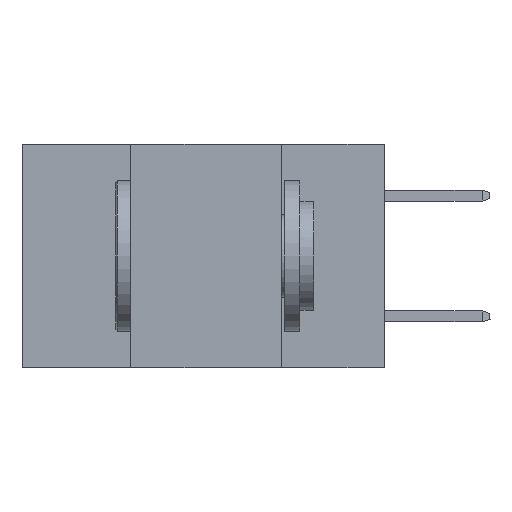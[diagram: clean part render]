
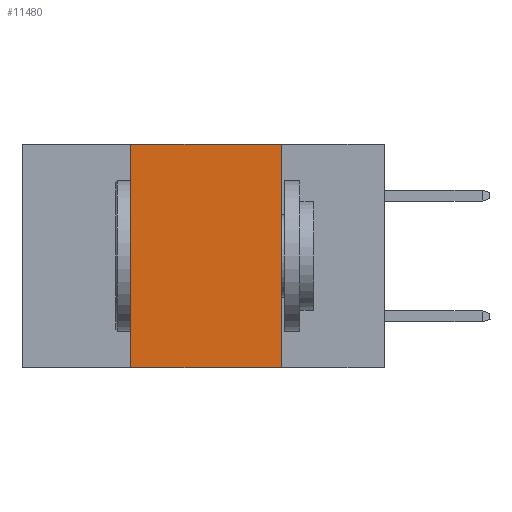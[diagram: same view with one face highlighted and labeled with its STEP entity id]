
A CAD part, left-side view. The second image highlights one B-rep face of the part: STEP entity #11480.
In plain terms, the highlighted planar face has unit normal (-1, 0, 0).
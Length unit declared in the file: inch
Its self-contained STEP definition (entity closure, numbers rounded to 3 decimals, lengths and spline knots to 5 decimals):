
#201 = CARTESIAN_POINT ( 'NONE',  ( 0., 0.17, -0.37 ) ) ;
#339 = AXIS2_PLACEMENT_3D ( 'NONE', #7886, #878, #10653 ) ;
#878 = DIRECTION ( 'NONE',  ( 1., 0., 0. ) ) ;
#1037 = CARTESIAN_POINT ( 'NONE',  ( 0., 0.17, 0. ) ) ;
#1873 = CARTESIAN_POINT ( 'NONE',  ( 0., 0.42, 0. ) ) ;
#2855 = FACE_OUTER_BOUND ( 'NONE', #5679, .T. ) ;
#2903 = VECTOR ( 'NONE', #10845, 39.37008 ) ;
#4138 = VERTEX_POINT ( 'NONE', #1873 ) ;
#4368 = VECTOR ( 'NONE', #5668, 39.37008 ) ;
#5668 = DIRECTION ( 'NONE',  ( 0., 0., 1. ) ) ;
#5679 = EDGE_LOOP ( 'NONE', ( #10128, #14899, #16560, #12497 ) ) ;
#5748 = EDGE_CURVE ( 'NONE', #11582, #15676, #6216, .T. ) ;
#6216 = LINE ( 'NONE', #9538, #13180 ) ;
#6492 = VERTEX_POINT ( 'NONE', #1037 ) ;
#6670 = EDGE_CURVE ( 'NONE', #11582, #4138, #8028, .T. ) ;
#6685 = CARTESIAN_POINT ( 'NONE',  ( 0., 0.42, -0.37 ) ) ;
#6703 = CARTESIAN_POINT ( 'NONE',  ( 0., 0.17, -0.37 ) ) ;
#7575 = EDGE_CURVE ( 'NONE', #4138, #6492, #15408, .T. ) ;
#7886 = CARTESIAN_POINT ( 'NONE',  ( 0., 0.6, 0. ) ) ;
#7994 = VECTOR ( 'NONE', #9496, 39.37008 ) ;
#8028 = LINE ( 'NONE', #11751, #4368 ) ;
#8197 = CARTESIAN_POINT ( 'NONE',  ( 0., 0.6, 0. ) ) ;
#9401 = EDGE_CURVE ( 'NONE', #6492, #15676, #14041, .T. ) ;
#9496 = DIRECTION ( 'NONE',  ( 0., -1., 0. ) ) ;
#9497 = DIRECTION ( 'NONE',  ( 0., -1., 0. ) ) ;
#9538 = CARTESIAN_POINT ( 'NONE',  ( 0., 0.6, -0.37 ) ) ;
#10128 = ORIENTED_EDGE ( 'NONE', *, *, #9401, .F. ) ;
#10653 = DIRECTION ( 'NONE',  ( 0., 0., -1. ) ) ;
#10845 = DIRECTION ( 'NONE',  ( 0., 0., -1. ) ) ;
#11480 = ADVANCED_FACE ( 'NONE', ( #2855 ), #16214, .F. ) ;
#11582 = VERTEX_POINT ( 'NONE', #6685 ) ;
#11751 = CARTESIAN_POINT ( 'NONE',  ( 0., 0.42, -0.37 ) ) ;
#12497 = ORIENTED_EDGE ( 'NONE', *, *, #5748, .T. ) ;
#13180 = VECTOR ( 'NONE', #9497, 39.37008 ) ;
#14041 = LINE ( 'NONE', #6703, #2903 ) ;
#14899 = ORIENTED_EDGE ( 'NONE', *, *, #7575, .F. ) ;
#15408 = LINE ( 'NONE', #8197, #7994 ) ;
#15676 = VERTEX_POINT ( 'NONE', #201 ) ;
#16214 = PLANE ( 'NONE',  #339 ) ;
#16560 = ORIENTED_EDGE ( 'NONE', *, *, #6670, .F. ) ;
